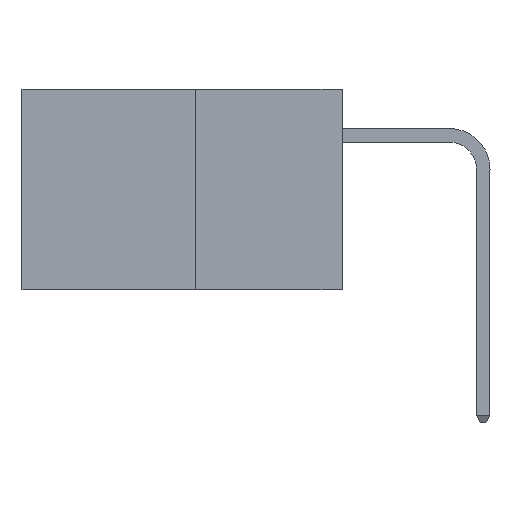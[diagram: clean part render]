
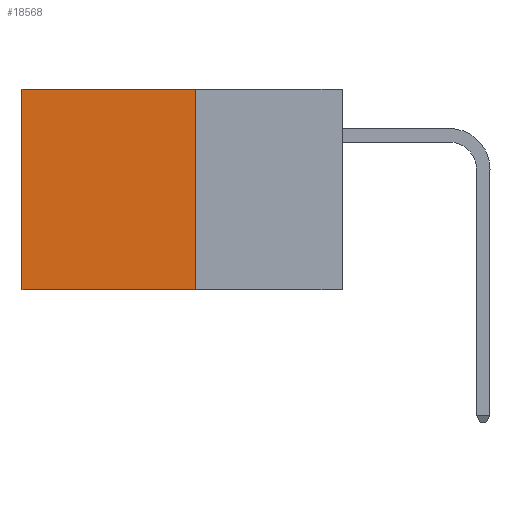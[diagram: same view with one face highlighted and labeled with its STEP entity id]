
A CAD part, left-side view. The second image highlights one B-rep face of the part: STEP entity #18568.
In plain terms, the highlighted planar face has unit normal (-1, 0, 0).
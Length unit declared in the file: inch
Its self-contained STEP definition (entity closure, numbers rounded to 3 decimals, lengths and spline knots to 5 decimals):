
#143 = VERTEX_POINT ( 'NONE', #9257 ) ;
#749 = AXIS2_PLACEMENT_3D ( 'NONE', #2640, #17217, #6325 ) ;
#1730 = LINE ( 'NONE', #10199, #15727 ) ;
#2640 = CARTESIAN_POINT ( 'NONE',  ( 0.277, 0.27, -0.37 ) ) ;
#3167 = FACE_OUTER_BOUND ( 'NONE', #13008, .T. ) ;
#3622 = ORIENTED_EDGE ( 'NONE', *, *, #12468, .F. ) ;
#3682 = LINE ( 'NONE', #18346, #12843 ) ;
#4463 = CARTESIAN_POINT ( 'NONE',  ( 0.277, 0.59, -0.37 ) ) ;
#5354 = VERTEX_POINT ( 'NONE', #20081 ) ;
#5466 = LINE ( 'NONE', #9952, #15142 ) ;
#6129 = EDGE_CURVE ( 'NONE', #13790, #143, #5466, .T. ) ;
#6325 = DIRECTION ( 'NONE',  ( 0., 0., -1. ) ) ;
#6373 = DIRECTION ( 'NONE',  ( 0., 0., -1. ) ) ;
#9257 = CARTESIAN_POINT ( 'NONE',  ( 0.277, 0.27, -0.37 ) ) ;
#9493 = VERTEX_POINT ( 'NONE', #16321 ) ;
#9779 = ORIENTED_EDGE ( 'NONE', *, *, #16070, .T. ) ;
#9952 = CARTESIAN_POINT ( 'NONE',  ( 0.277, 0.27, -0.37 ) ) ;
#10199 = CARTESIAN_POINT ( 'NONE',  ( 0.277, 0.27, 0. ) ) ;
#11045 = CARTESIAN_POINT ( 'NONE',  ( 0.277, 0.27, 0. ) ) ;
#11186 = DIRECTION ( 'NONE',  ( 0., 1., 0. ) ) ;
#11758 = PLANE ( 'NONE',  #749 ) ;
#12468 = EDGE_CURVE ( 'NONE', #143, #9493, #3682, .T. ) ;
#12843 = VECTOR ( 'NONE', #11186, 39.37008 ) ;
#13008 = EDGE_LOOP ( 'NONE', ( #14735, #3622, #17171, #9779 ) ) ;
#13790 = VERTEX_POINT ( 'NONE', #11045 ) ;
#13851 = DIRECTION ( 'NONE',  ( 0., 1., 0. ) ) ;
#14735 = ORIENTED_EDGE ( 'NONE', *, *, #19617, .T. ) ;
#15142 = VECTOR ( 'NONE', #22524, 39.37008 ) ;
#15727 = VECTOR ( 'NONE', #13851, 39.37008 ) ;
#16070 = EDGE_CURVE ( 'NONE', #13790, #5354, #1730, .T. ) ;
#16321 = CARTESIAN_POINT ( 'NONE',  ( 0.277, 0.59, -0.37 ) ) ;
#17171 = ORIENTED_EDGE ( 'NONE', *, *, #6129, .F. ) ;
#17217 = DIRECTION ( 'NONE',  ( 1., 0., 0. ) ) ;
#17342 = VECTOR ( 'NONE', #6373, 39.37008 ) ;
#17903 = LINE ( 'NONE', #4463, #17342 ) ;
#18346 = CARTESIAN_POINT ( 'NONE',  ( 0.277, 0.27, -0.37 ) ) ;
#18568 = ADVANCED_FACE ( 'NONE', ( #3167 ), #11758, .F. ) ;
#19617 = EDGE_CURVE ( 'NONE', #5354, #9493, #17903, .T. ) ;
#20081 = CARTESIAN_POINT ( 'NONE',  ( 0.277, 0.59, 0. ) ) ;
#22524 = DIRECTION ( 'NONE',  ( 0., 0., -1. ) ) ;
